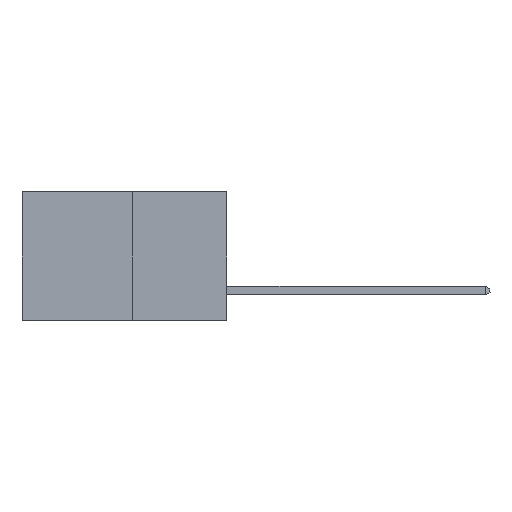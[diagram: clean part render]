
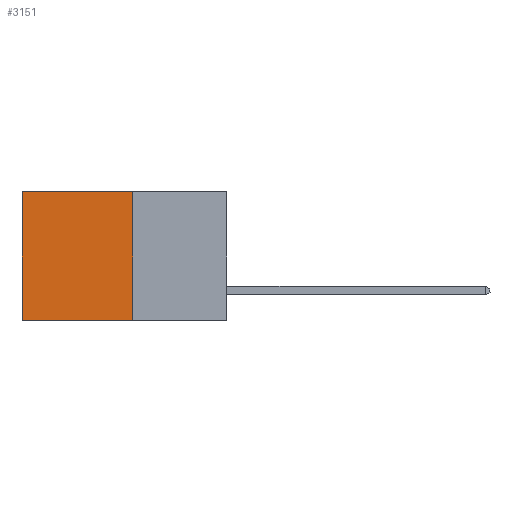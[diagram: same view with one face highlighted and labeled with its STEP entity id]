
A CAD part, left-side view. The second image highlights one B-rep face of the part: STEP entity #3151.
In plain terms, the highlighted planar face has unit normal (-1, 0, 0).
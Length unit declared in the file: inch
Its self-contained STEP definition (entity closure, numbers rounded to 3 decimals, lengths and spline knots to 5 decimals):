
#254 = DIRECTION ( 'NONE',  ( 0., 1., 0. ) ) ;
#789 = VERTEX_POINT ( 'NONE', #3536 ) ;
#1392 = DIRECTION ( 'NONE',  ( 0., 0., -1. ) ) ;
#1430 = VERTEX_POINT ( 'NONE', #7938 ) ;
#1969 = ORIENTED_EDGE ( 'NONE', *, *, #5470, .T. ) ;
#2043 = ORIENTED_EDGE ( 'NONE', *, *, #4380, .F. ) ;
#2574 = VERTEX_POINT ( 'NONE', #3428 ) ;
#2691 = EDGE_LOOP ( 'NONE', ( #1969, #3482, #2043, #7932 ) ) ;
#2805 = VECTOR ( 'NONE', #9593, 39.37008 ) ;
#3151 = ADVANCED_FACE ( 'NONE', ( #4394 ), #15145, .F. ) ;
#3428 = CARTESIAN_POINT ( 'NONE',  ( 0.277, 0.59, 0. ) ) ;
#3482 = ORIENTED_EDGE ( 'NONE', *, *, #8237, .F. ) ;
#3536 = CARTESIAN_POINT ( 'NONE',  ( 0.277, 0.27, -0.37 ) ) ;
#4380 = EDGE_CURVE ( 'NONE', #1430, #789, #9035, .T. ) ;
#4394 = FACE_OUTER_BOUND ( 'NONE', #2691, .T. ) ;
#4621 = LINE ( 'NONE', #8631, #7094 ) ;
#4987 = DIRECTION ( 'NONE',  ( 0., 1., 0. ) ) ;
#5012 = LINE ( 'NONE', #11079, #11023 ) ;
#5470 = EDGE_CURVE ( 'NONE', #2574, #13011, #9195, .T. ) ;
#7094 = VECTOR ( 'NONE', #4987, 39.37008 ) ;
#7743 = EDGE_CURVE ( 'NONE', #1430, #2574, #5012, .T. ) ;
#7932 = ORIENTED_EDGE ( 'NONE', *, *, #7743, .T. ) ;
#7938 = CARTESIAN_POINT ( 'NONE',  ( 0.277, 0.27, 0. ) ) ;
#8237 = EDGE_CURVE ( 'NONE', #789, #13011, #4621, .T. ) ;
#8628 = CARTESIAN_POINT ( 'NONE',  ( 0.277, 0.27, -0.37 ) ) ;
#8631 = CARTESIAN_POINT ( 'NONE',  ( 0.277, 0.27, -0.37 ) ) ;
#9035 = LINE ( 'NONE', #8628, #11820 ) ;
#9195 = LINE ( 'NONE', #9653, #2805 ) ;
#9593 = DIRECTION ( 'NONE',  ( 0., 0., -1. ) ) ;
#9653 = CARTESIAN_POINT ( 'NONE',  ( 0.277, 0.59, -0.37 ) ) ;
#9857 = AXIS2_PLACEMENT_3D ( 'NONE', #12776, #12190, #11475 ) ;
#11023 = VECTOR ( 'NONE', #254, 39.37008 ) ;
#11079 = CARTESIAN_POINT ( 'NONE',  ( 0.277, 0.27, 0. ) ) ;
#11424 = CARTESIAN_POINT ( 'NONE',  ( 0.277, 0.59, -0.37 ) ) ;
#11475 = DIRECTION ( 'NONE',  ( 0., 0., -1. ) ) ;
#11820 = VECTOR ( 'NONE', #1392, 39.37008 ) ;
#12190 = DIRECTION ( 'NONE',  ( 1., 0., 0. ) ) ;
#12776 = CARTESIAN_POINT ( 'NONE',  ( 0.277, 0.27, -0.37 ) ) ;
#13011 = VERTEX_POINT ( 'NONE', #11424 ) ;
#15145 = PLANE ( 'NONE',  #9857 ) ;
